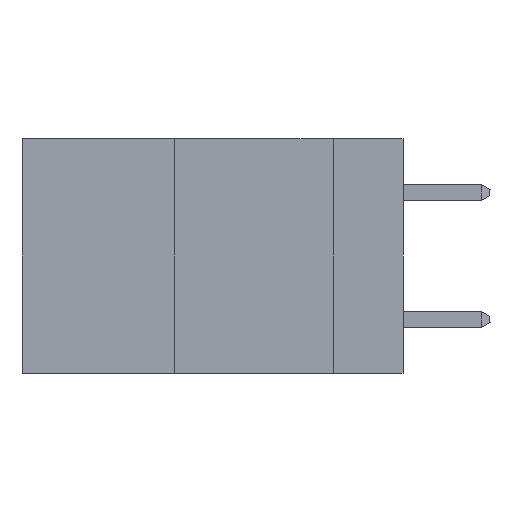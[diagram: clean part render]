
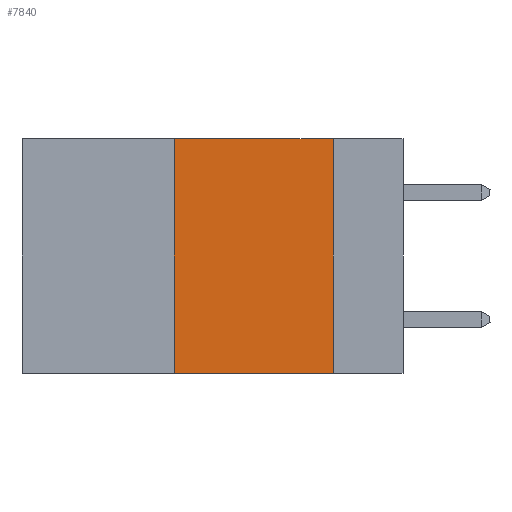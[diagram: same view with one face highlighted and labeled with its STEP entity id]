
A CAD part, left-side view. The second image highlights one B-rep face of the part: STEP entity #7840.
In plain terms, the highlighted planar face has unit normal (-1, 0, 0).
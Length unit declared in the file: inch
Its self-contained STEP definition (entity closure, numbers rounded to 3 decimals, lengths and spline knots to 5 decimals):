
#507 = CARTESIAN_POINT ( 'NONE',  ( 0., 0.36, 0. ) ) ;
#594 = EDGE_CURVE ( 'NONE', #1757, #5781, #12356, .T. ) ;
#892 = CARTESIAN_POINT ( 'NONE',  ( 0., 0.6, 0. ) ) ;
#1308 = VERTEX_POINT ( 'NONE', #33355 ) ;
#1757 = VERTEX_POINT ( 'NONE', #26253 ) ;
#2566 = CARTESIAN_POINT ( 'NONE',  ( 0., 0.11, -0.37 ) ) ;
#3965 = DIRECTION ( 'NONE',  ( 0., -1., 0. ) ) ;
#4341 = LINE ( 'NONE', #892, #19351 ) ;
#5781 = VERTEX_POINT ( 'NONE', #507 ) ;
#7840 = ADVANCED_FACE ( 'NONE', ( #37338 ), #11941, .F. ) ;
#8611 = DIRECTION ( 'NONE',  ( 0., 0., 1. ) ) ;
#8728 = CARTESIAN_POINT ( 'NONE',  ( 0., 0.36, 0. ) ) ;
#10075 = EDGE_CURVE ( 'NONE', #5781, #1308, #4341, .T. ) ;
#11941 = PLANE ( 'NONE',  #26829 ) ;
#12356 = LINE ( 'NONE', #8728, #21302 ) ;
#17932 = DIRECTION ( 'NONE',  ( 0., 0., -1. ) ) ;
#19351 = VECTOR ( 'NONE', #3965, 39.37008 ) ;
#21302 = VECTOR ( 'NONE', #8611, 39.37008 ) ;
#21977 = ORIENTED_EDGE ( 'NONE', *, *, #31073, .F. ) ;
#22527 = CARTESIAN_POINT ( 'NONE',  ( 0., 0.6, -0.37 ) ) ;
#22871 = ORIENTED_EDGE ( 'NONE', *, *, #10075, .F. ) ;
#23095 = ORIENTED_EDGE ( 'NONE', *, *, #594, .F. ) ;
#23520 = CARTESIAN_POINT ( 'NONE',  ( 0., 0.11, 0. ) ) ;
#24883 = VECTOR ( 'NONE', #26521, 39.37008 ) ;
#25501 = ORIENTED_EDGE ( 'NONE', *, *, #27878, .T. ) ;
#26253 = CARTESIAN_POINT ( 'NONE',  ( 0., 0.36, -0.37 ) ) ;
#26521 = DIRECTION ( 'NONE',  ( 0., 0., -1. ) ) ;
#26829 = AXIS2_PLACEMENT_3D ( 'NONE', #32955, #35911, #17932 ) ;
#27878 = EDGE_CURVE ( 'NONE', #1757, #35039, #28216, .T. ) ;
#28216 = LINE ( 'NONE', #22527, #35239 ) ;
#31073 = EDGE_CURVE ( 'NONE', #1308, #35039, #32838, .T. ) ;
#31572 = DIRECTION ( 'NONE',  ( 0., -1., 0. ) ) ;
#32814 = EDGE_LOOP ( 'NONE', ( #21977, #22871, #23095, #25501 ) ) ;
#32838 = LINE ( 'NONE', #23520, #24883 ) ;
#32955 = CARTESIAN_POINT ( 'NONE',  ( 0., 0.6, 0. ) ) ;
#33355 = CARTESIAN_POINT ( 'NONE',  ( 0., 0.11, 0. ) ) ;
#35039 = VERTEX_POINT ( 'NONE', #2566 ) ;
#35239 = VECTOR ( 'NONE', #31572, 39.37008 ) ;
#35911 = DIRECTION ( 'NONE',  ( 1., 0., 0. ) ) ;
#37338 = FACE_OUTER_BOUND ( 'NONE', #32814, .T. ) ;
